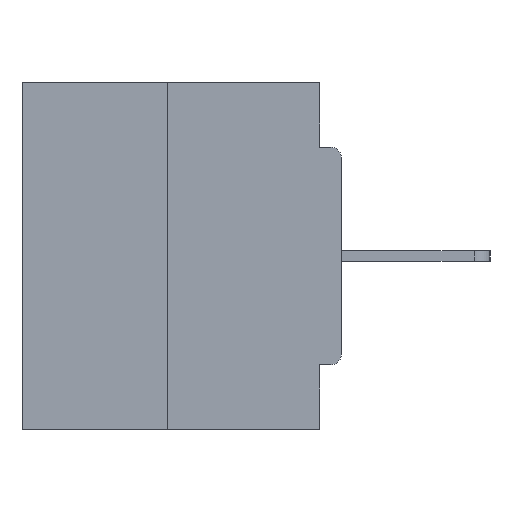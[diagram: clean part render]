
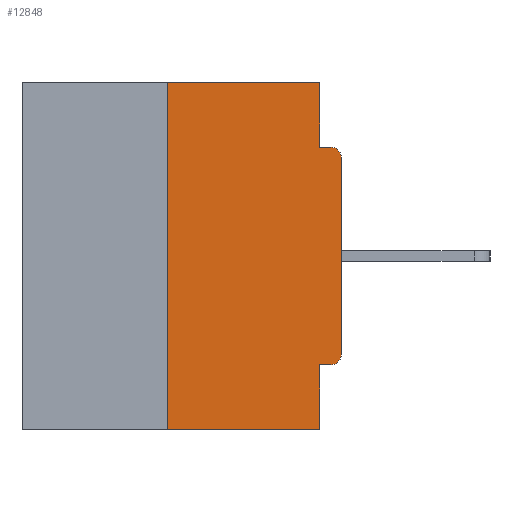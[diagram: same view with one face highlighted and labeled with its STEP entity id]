
A CAD part, left-side view. The second image highlights one B-rep face of the part: STEP entity #12848.
In plain terms, the highlighted planar face has unit normal (-1, 0, 0).
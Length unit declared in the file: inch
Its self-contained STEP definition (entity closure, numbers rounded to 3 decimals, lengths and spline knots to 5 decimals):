
#206 = VERTEX_POINT ( 'NONE', #20777 ) ;
#919 = VECTOR ( 'NONE', #4267, 39.37008 ) ;
#988 = EDGE_CURVE ( 'NONE', #11546, #28714, #24434, .T. ) ;
#1058 = ORIENTED_EDGE ( 'NONE', *, *, #27184, .F. ) ;
#1283 = VERTEX_POINT ( 'NONE', #25086 ) ;
#1657 = ORIENTED_EDGE ( 'NONE', *, *, #11966, .F. ) ;
#1720 = ORIENTED_EDGE ( 'NONE', *, *, #4729, .T. ) ;
#1887 = VERTEX_POINT ( 'NONE', #23140 ) ;
#1890 = CARTESIAN_POINT ( 'NONE',  ( 0., 0., -0.1085 ) ) ;
#2090 = VECTOR ( 'NONE', #27990, 39.37008 ) ;
#2550 = CARTESIAN_POINT ( 'NONE',  ( 0., 0.46, -0.5 ) ) ;
#2576 = ORIENTED_EDGE ( 'NONE', *, *, #2859, .F. ) ;
#2859 = EDGE_CURVE ( 'NONE', #1283, #206, #26351, .T. ) ;
#3152 = ORIENTED_EDGE ( 'NONE', *, *, #18205, .F. ) ;
#3391 = ORIENTED_EDGE ( 'NONE', *, *, #29617, .T. ) ;
#3561 = DIRECTION ( 'NONE',  ( 0., -1., 0. ) ) ;
#3842 = ORIENTED_EDGE ( 'NONE', *, *, #8647, .T. ) ;
#3939 = ORIENTED_EDGE ( 'NONE', *, *, #26049, .T. ) ;
#4057 = ORIENTED_EDGE ( 'NONE', *, *, #5668, .F. ) ;
#4267 = DIRECTION ( 'NONE',  ( 0., -1., 0. ) ) ;
#4649 = ORIENTED_EDGE ( 'NONE', *, *, #988, .F. ) ;
#4715 = CARTESIAN_POINT ( 'NONE',  ( 0., 0.015, -0.3915 ) ) ;
#4729 = EDGE_CURVE ( 'NONE', #29393, #206, #25031, .T. ) ;
#4827 = AXIS2_PLACEMENT_3D ( 'NONE', #30942, #12713, #31285 ) ;
#5131 = AXIS2_PLACEMENT_3D ( 'NONE', #6924, #25629, #9680 ) ;
#5585 = VECTOR ( 'NONE', #11954, 39.37008 ) ;
#5668 = EDGE_CURVE ( 'NONE', #28714, #6800, #8263, .T. ) ;
#6347 = CARTESIAN_POINT ( 'NONE',  ( 0., 0., -0.0935 ) ) ;
#6800 = VERTEX_POINT ( 'NONE', #9411 ) ;
#6924 = CARTESIAN_POINT ( 'NONE',  ( 0., 0.015, -0.1085 ) ) ;
#7445 = DIRECTION ( 'NONE',  ( 0., 0., -1. ) ) ;
#8263 = LINE ( 'NONE', #6347, #919 ) ;
#8289 = CARTESIAN_POINT ( 'NONE',  ( 0., 0.25, 0. ) ) ;
#8305 = DIRECTION ( 'NONE',  ( 0., 0., 1. ) ) ;
#8647 = EDGE_CURVE ( 'NONE', #22637, #32919, #29130, .T. ) ;
#8806 = CIRCLE ( 'NONE', #20474, 0.015 ) ;
#8891 = EDGE_LOOP ( 'NONE', ( #1058, #1657, #1720, #2576, #3152, #3391, #3842, #3939, #4057, #4649 ) ) ;
#9339 = FACE_OUTER_BOUND ( 'NONE', #8891, .T. ) ;
#9411 = CARTESIAN_POINT ( 'NONE',  ( 0., 0.015, -0.0935 ) ) ;
#9680 = DIRECTION ( 'NONE',  ( 0., 0., -1. ) ) ;
#11546 = VERTEX_POINT ( 'NONE', #16433 ) ;
#11954 = DIRECTION ( 'NONE',  ( 0., -1., 0. ) ) ;
#11966 = EDGE_CURVE ( 'NONE', #29393, #18927, #13104, .T. ) ;
#12713 = DIRECTION ( 'NONE',  ( 1., 0., 0. ) ) ;
#12750 = LINE ( 'NONE', #30526, #5585 ) ;
#12848 = ADVANCED_FACE ( 'NONE', ( #9339 ), #28665, .F. ) ;
#13104 = LINE ( 'NONE', #8289, #19342 ) ;
#13175 = CARTESIAN_POINT ( 'NONE',  ( 0., 0.25, 0. ) ) ;
#13606 = CARTESIAN_POINT ( 'NONE',  ( 0., 0., -0.3915 ) ) ;
#14119 = VECTOR ( 'NONE', #20114, 39.37008 ) ;
#15042 = DIRECTION ( 'NONE',  ( 0., 1., 0. ) ) ;
#15772 = DIRECTION ( 'NONE',  ( 0., 0., -1. ) ) ;
#16433 = CARTESIAN_POINT ( 'NONE',  ( 0., 0.031, 0. ) ) ;
#17586 = CARTESIAN_POINT ( 'NONE',  ( 0., 0., -0.4065 ) ) ;
#17880 = VECTOR ( 'NONE', #3561, 39.37008 ) ;
#18205 = EDGE_CURVE ( 'NONE', #1887, #1283, #34717, .T. ) ;
#18394 = VECTOR ( 'NONE', #15772, 39.37008 ) ;
#18927 = VERTEX_POINT ( 'NONE', #13175 ) ;
#19342 = VECTOR ( 'NONE', #8305, 39.37008 ) ;
#19823 = CARTESIAN_POINT ( 'NONE',  ( 0., 0.031, -0.5 ) ) ;
#20114 = DIRECTION ( 'NONE',  ( 0., 0., 1. ) ) ;
#20301 = CARTESIAN_POINT ( 'NONE',  ( 0., 0., 0. ) ) ;
#20474 = AXIS2_PLACEMENT_3D ( 'NONE', #4715, #23469, #7445 ) ;
#20777 = CARTESIAN_POINT ( 'NONE',  ( 0., 0.031, -0.5 ) ) ;
#21853 = CARTESIAN_POINT ( 'NONE',  ( 0., 0.25, -0.5 ) ) ;
#22637 = VERTEX_POINT ( 'NONE', #13606 ) ;
#23140 = CARTESIAN_POINT ( 'NONE',  ( 0., 0.015, -0.4065 ) ) ;
#23469 = DIRECTION ( 'NONE',  ( -1., 0., 0. ) ) ;
#24434 = LINE ( 'NONE', #32349, #2090 ) ;
#25031 = LINE ( 'NONE', #2550, #17880 ) ;
#25086 = CARTESIAN_POINT ( 'NONE',  ( 0., 0.031, -0.4065 ) ) ;
#25629 = DIRECTION ( 'NONE',  ( -1., 0., 0. ) ) ;
#26049 = EDGE_CURVE ( 'NONE', #32919, #6800, #29089, .T. ) ;
#26351 = LINE ( 'NONE', #19823, #18394 ) ;
#27184 = EDGE_CURVE ( 'NONE', #18927, #11546, #12750, .T. ) ;
#27752 = VECTOR ( 'NONE', #15042, 39.37008 ) ;
#27990 = DIRECTION ( 'NONE',  ( 0., 0., -1. ) ) ;
#28665 = PLANE ( 'NONE',  #4827 ) ;
#28714 = VERTEX_POINT ( 'NONE', #34691 ) ;
#29089 = CIRCLE ( 'NONE', #5131, 0.015 ) ;
#29130 = LINE ( 'NONE', #20301, #14119 ) ;
#29393 = VERTEX_POINT ( 'NONE', #21853 ) ;
#29617 = EDGE_CURVE ( 'NONE', #1887, #22637, #8806, .T. ) ;
#30526 = CARTESIAN_POINT ( 'NONE',  ( 0., 0.46, 0. ) ) ;
#30942 = CARTESIAN_POINT ( 'NONE',  ( 0., 0.46, 0. ) ) ;
#31285 = DIRECTION ( 'NONE',  ( 0., 0., -1. ) ) ;
#32349 = CARTESIAN_POINT ( 'NONE',  ( 0., 0.031, 0. ) ) ;
#32919 = VERTEX_POINT ( 'NONE', #1890 ) ;
#34691 = CARTESIAN_POINT ( 'NONE',  ( 0., 0.031, -0.0935 ) ) ;
#34717 = LINE ( 'NONE', #17586, #27752 ) ;
